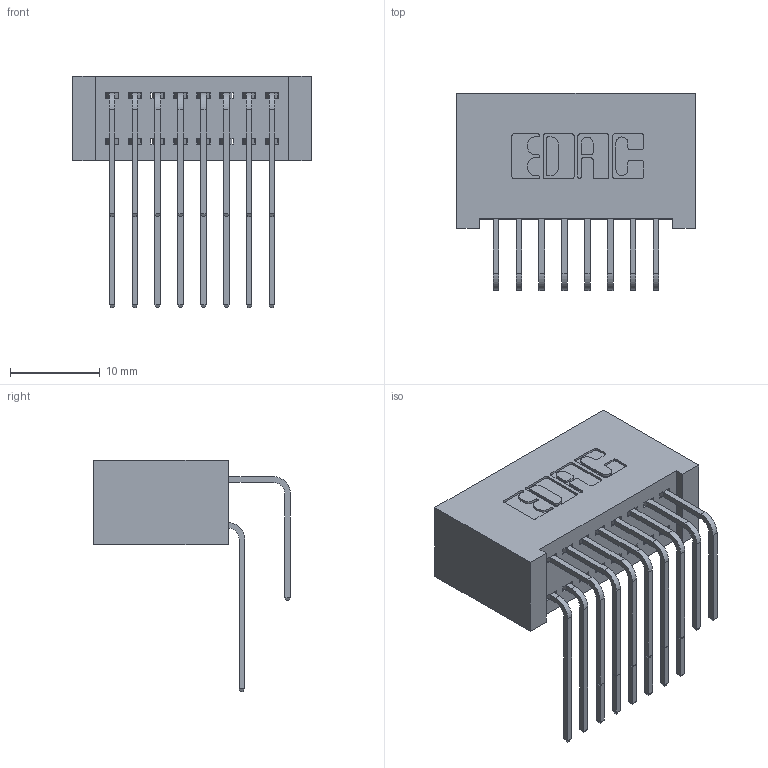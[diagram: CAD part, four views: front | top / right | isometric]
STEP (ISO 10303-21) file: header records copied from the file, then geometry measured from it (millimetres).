
FILE_DESCRIPTION (( 'STEP AP203' ), '1' );
FILE_NAME ('392-016-558-201.STEP', '2019-10-07T03:26:25', ( '' ), ( '' ), 'SwSTEP 2.0', 'SolidWorks 2016', '' );
FILE_SCHEMA (( 'CONFIG_CONTROL_DESIGN' ));
Length unit declared in the file: inch
Products named in the file (4): 345-292-001_558 Tail - 2; 392-016-558-201; 342 Part_Lugless; 345-292-001_558 559 Tail - 1
Assembly tree (17 placements, depth 2):
  392-016-558-201
    342 Part_Lugless
    345-292-001_558 559 Tail - 1  x8
    345-292-001_558 Tail - 2  x8
Bounding box: 26.57 x 21.91 x 25.78 mm (x, y, z)
Volume: 2758 mm3; surface area: 4515.4 mm2
Topology: 17 solids, 17 shells, 966 faces, 2851 edges, 1878 vertices
Faces by surface type: plane 670, cylinder 296
Entity records: 10919 total; most frequent: CARTESIAN_POINT 1897, ORIENTED_EDGE 1782, DIRECTION 1655, EDGE_CURVE 891, VECTOR 731, LINE 731, VERTEX_POINT 590, AXIS2_PLACEMENT_3D 462
